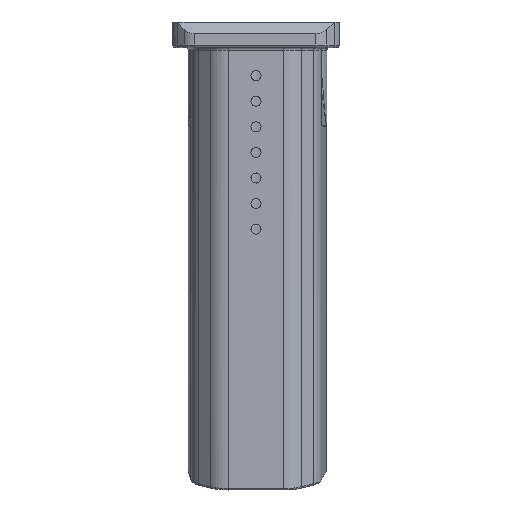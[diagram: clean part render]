
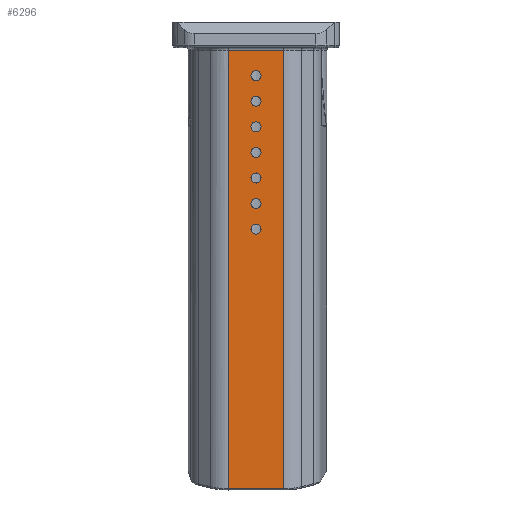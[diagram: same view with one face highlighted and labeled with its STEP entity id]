
A CAD part, front view. The second image highlights one B-rep face of the part: STEP entity #6296.
In plain terms, the highlighted planar face has unit normal (0, -1, 0).
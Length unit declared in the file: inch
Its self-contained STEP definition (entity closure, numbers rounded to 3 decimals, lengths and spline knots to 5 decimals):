
#50=FACE_BOUND('',#1745,.T.);
#51=FACE_BOUND('',#1746,.T.);
#52=FACE_BOUND('',#1747,.T.);
#53=FACE_BOUND('',#1748,.T.);
#54=FACE_BOUND('',#1749,.T.);
#55=FACE_BOUND('',#1750,.T.);
#56=FACE_BOUND('',#1751,.T.);
#136=PLANE('',#6984);
#452=LINE('',#13276,#797);
#485=LINE('',#13548,#830);
#486=LINE('',#13552,#831);
#515=LINE('',#14260,#860);
#797=VECTOR('',#8182,39.37008);
#830=VECTOR('',#8371,39.37008);
#831=VECTOR('',#8376,39.37008);
#860=VECTOR('',#8463,39.37008);
#1344=FACE_OUTER_BOUND('',#1744,.T.);
#1744=EDGE_LOOP('',(#5318,#5319,#5320,#5321));
#1745=EDGE_LOOP('',(#5322,#5323));
#1746=EDGE_LOOP('',(#5324,#5325));
#1747=EDGE_LOOP('',(#5326,#5327));
#1748=EDGE_LOOP('',(#5328,#5329));
#1749=EDGE_LOOP('',(#5330,#5331));
#1750=EDGE_LOOP('',(#5332,#5333));
#1751=EDGE_LOOP('',(#5334,#5335));
#2099=CIRCLE('',#6792,0.09843);
#2100=CIRCLE('',#6793,0.09843);
#2102=CIRCLE('',#6796,0.09843);
#2103=CIRCLE('',#6797,0.09843);
#2105=CIRCLE('',#6800,0.09843);
#2106=CIRCLE('',#6801,0.09843);
#2108=CIRCLE('',#6804,0.09843);
#2109=CIRCLE('',#6805,0.09843);
#2112=CIRCLE('',#6810,0.09843);
#2113=CIRCLE('',#6811,0.09843);
#2115=CIRCLE('',#6814,0.09843);
#2116=CIRCLE('',#6815,0.09843);
#2118=CIRCLE('',#6818,0.09843);
#2119=CIRCLE('',#6819,0.09843);
#2880=VERTEX_POINT('',#12572);
#2881=VERTEX_POINT('',#12573);
#2883=VERTEX_POINT('',#12580);
#2884=VERTEX_POINT('',#12581);
#2886=VERTEX_POINT('',#12588);
#2887=VERTEX_POINT('',#12589);
#2889=VERTEX_POINT('',#12596);
#2890=VERTEX_POINT('',#12597);
#2894=VERTEX_POINT('',#12608);
#2895=VERTEX_POINT('',#12609);
#2897=VERTEX_POINT('',#12616);
#2898=VERTEX_POINT('',#12617);
#2900=VERTEX_POINT('',#12624);
#2901=VERTEX_POINT('',#12625);
#2956=VERTEX_POINT('',#13272);
#2957=VERTEX_POINT('',#13274);
#3006=VERTEX_POINT('',#13546);
#3007=VERTEX_POINT('',#13551);
#3631=EDGE_CURVE('',#2880,#2881,#2099,.T.);
#3632=EDGE_CURVE('',#2881,#2880,#2100,.T.);
#3635=EDGE_CURVE('',#2883,#2884,#2102,.T.);
#3636=EDGE_CURVE('',#2884,#2883,#2103,.T.);
#3639=EDGE_CURVE('',#2886,#2887,#2105,.T.);
#3640=EDGE_CURVE('',#2887,#2886,#2106,.T.);
#3643=EDGE_CURVE('',#2889,#2890,#2108,.T.);
#3644=EDGE_CURVE('',#2890,#2889,#2109,.T.);
#3649=EDGE_CURVE('',#2894,#2895,#2112,.T.);
#3650=EDGE_CURVE('',#2895,#2894,#2113,.T.);
#3653=EDGE_CURVE('',#2897,#2898,#2115,.T.);
#3654=EDGE_CURVE('',#2898,#2897,#2116,.T.);
#3657=EDGE_CURVE('',#2900,#2901,#2118,.T.);
#3658=EDGE_CURVE('',#2901,#2900,#2119,.T.);
#3748=EDGE_CURVE('',#2957,#2956,#452,.T.);
#3836=EDGE_CURVE('',#2957,#3006,#485,.T.);
#3838=EDGE_CURVE('',#2956,#3007,#486,.T.);
#3894=EDGE_CURVE('',#3006,#3007,#515,.T.);
#5318=ORIENTED_EDGE('',*,*,#3836,.T.);
#5319=ORIENTED_EDGE('',*,*,#3894,.T.);
#5320=ORIENTED_EDGE('',*,*,#3838,.F.);
#5321=ORIENTED_EDGE('',*,*,#3748,.F.);
#5322=ORIENTED_EDGE('',*,*,#3631,.T.);
#5323=ORIENTED_EDGE('',*,*,#3632,.T.);
#5324=ORIENTED_EDGE('',*,*,#3635,.T.);
#5325=ORIENTED_EDGE('',*,*,#3636,.T.);
#5326=ORIENTED_EDGE('',*,*,#3639,.T.);
#5327=ORIENTED_EDGE('',*,*,#3640,.T.);
#5328=ORIENTED_EDGE('',*,*,#3643,.T.);
#5329=ORIENTED_EDGE('',*,*,#3644,.T.);
#5330=ORIENTED_EDGE('',*,*,#3649,.T.);
#5331=ORIENTED_EDGE('',*,*,#3650,.T.);
#5332=ORIENTED_EDGE('',*,*,#3653,.T.);
#5333=ORIENTED_EDGE('',*,*,#3654,.T.);
#5334=ORIENTED_EDGE('',*,*,#3657,.T.);
#5335=ORIENTED_EDGE('',*,*,#3658,.T.);
#6296=ADVANCED_FACE('',(#1344,#50,#51,#52,#53,#54,#55,#56),#136,.T.);
#6792=AXIS2_PLACEMENT_3D('',#12574,#7985,#7986);
#6793=AXIS2_PLACEMENT_3D('',#12575,#7987,#7988);
#6796=AXIS2_PLACEMENT_3D('',#12582,#7994,#7995);
#6797=AXIS2_PLACEMENT_3D('',#12583,#7996,#7997);
#6800=AXIS2_PLACEMENT_3D('',#12590,#8003,#8004);
#6801=AXIS2_PLACEMENT_3D('',#12591,#8005,#8006);
#6804=AXIS2_PLACEMENT_3D('',#12598,#8012,#8013);
#6805=AXIS2_PLACEMENT_3D('',#12599,#8014,#8015);
#6810=AXIS2_PLACEMENT_3D('',#12610,#8025,#8026);
#6811=AXIS2_PLACEMENT_3D('',#12611,#8027,#8028);
#6814=AXIS2_PLACEMENT_3D('',#12618,#8034,#8035);
#6815=AXIS2_PLACEMENT_3D('',#12619,#8036,#8037);
#6818=AXIS2_PLACEMENT_3D('',#12626,#8043,#8044);
#6819=AXIS2_PLACEMENT_3D('',#12627,#8045,#8046);
#6984=AXIS2_PLACEMENT_3D('',#14259,#8461,#8462);
#7985=DIRECTION('center_axis',(0.,1.,0.));
#7986=DIRECTION('ref_axis',(1.,0.,0.));
#7987=DIRECTION('center_axis',(0.,1.,0.));
#7988=DIRECTION('ref_axis',(1.,0.,0.));
#7994=DIRECTION('center_axis',(0.,1.,0.));
#7995=DIRECTION('ref_axis',(1.,0.,0.));
#7996=DIRECTION('center_axis',(0.,1.,0.));
#7997=DIRECTION('ref_axis',(1.,0.,0.));
#8003=DIRECTION('center_axis',(0.,1.,0.));
#8004=DIRECTION('ref_axis',(1.,0.,0.));
#8005=DIRECTION('center_axis',(0.,1.,0.));
#8006=DIRECTION('ref_axis',(1.,0.,0.));
#8012=DIRECTION('center_axis',(0.,1.,0.));
#8013=DIRECTION('ref_axis',(1.,0.,0.));
#8014=DIRECTION('center_axis',(0.,1.,0.));
#8015=DIRECTION('ref_axis',(1.,0.,0.));
#8025=DIRECTION('center_axis',(0.,1.,0.));
#8026=DIRECTION('ref_axis',(1.,0.,0.));
#8027=DIRECTION('center_axis',(0.,1.,0.));
#8028=DIRECTION('ref_axis',(1.,0.,0.));
#8034=DIRECTION('center_axis',(0.,1.,0.));
#8035=DIRECTION('ref_axis',(1.,0.,0.));
#8036=DIRECTION('center_axis',(0.,1.,0.));
#8037=DIRECTION('ref_axis',(1.,0.,0.));
#8043=DIRECTION('center_axis',(0.,1.,0.));
#8044=DIRECTION('ref_axis',(1.,0.,0.));
#8045=DIRECTION('center_axis',(0.,1.,0.));
#8046=DIRECTION('ref_axis',(1.,0.,0.));
#8182=DIRECTION('',(1.,0.,0.));
#8371=DIRECTION('',(0.,0.,-1.));
#8376=DIRECTION('',(0.,0.,-1.));
#8461=DIRECTION('center_axis',(0.,-1.,0.));
#8462=DIRECTION('ref_axis',(0.,0.,-1.));
#8463=DIRECTION('',(1.,0.,0.));
#12572=CARTESIAN_POINT('',(4.51516,-0.4932,-1.55));
#12573=CARTESIAN_POINT('',(4.31831,-0.4932,-1.55));
#12574=CARTESIAN_POINT('Origin',(4.41673,-0.4932,-1.55));
#12575=CARTESIAN_POINT('Origin',(4.41673,-0.4932,-1.55));
#12580=CARTESIAN_POINT('',(4.51516,-0.4932,-3.55));
#12581=CARTESIAN_POINT('',(4.31831,-0.4932,-3.55));
#12582=CARTESIAN_POINT('Origin',(4.41673,-0.4932,-3.55));
#12583=CARTESIAN_POINT('Origin',(4.41673,-0.4932,-3.55));
#12588=CARTESIAN_POINT('',(4.51516,-0.4932,-2.05));
#12589=CARTESIAN_POINT('',(4.31831,-0.4932,-2.05));
#12590=CARTESIAN_POINT('Origin',(4.41673,-0.4932,-2.05));
#12591=CARTESIAN_POINT('Origin',(4.41673,-0.4932,-2.05));
#12596=CARTESIAN_POINT('',(4.51516,-0.4932,-1.05));
#12597=CARTESIAN_POINT('',(4.31831,-0.4932,-1.05));
#12598=CARTESIAN_POINT('Origin',(4.41673,-0.4932,-1.05));
#12599=CARTESIAN_POINT('Origin',(4.41673,-0.4932,-1.05));
#12608=CARTESIAN_POINT('',(4.51516,-0.4932,-3.05));
#12609=CARTESIAN_POINT('',(4.31831,-0.4932,-3.05));
#12610=CARTESIAN_POINT('Origin',(4.41673,-0.4932,-3.05));
#12611=CARTESIAN_POINT('Origin',(4.41673,-0.4932,-3.05));
#12616=CARTESIAN_POINT('',(4.51516,-0.4932,-2.55));
#12617=CARTESIAN_POINT('',(4.31831,-0.4932,-2.55));
#12618=CARTESIAN_POINT('Origin',(4.41673,-0.4932,-2.55));
#12619=CARTESIAN_POINT('Origin',(4.41673,-0.4932,-2.55));
#12624=CARTESIAN_POINT('',(4.51516,-0.4932,-0.55));
#12625=CARTESIAN_POINT('',(4.31831,-0.4932,-0.55));
#12626=CARTESIAN_POINT('Origin',(4.41673,-0.4932,-0.55));
#12627=CARTESIAN_POINT('Origin',(4.41673,-0.4932,-0.55));
#13272=CARTESIAN_POINT('',(4.95505,-0.4932,-0.05));
#13274=CARTESIAN_POINT('',(3.87842,-0.4932,-0.05));
#13276=CARTESIAN_POINT('',(4.78942,-0.4932,-0.05));
#13546=CARTESIAN_POINT('',(3.87842,-0.4932,-8.62159));
#13548=CARTESIAN_POINT('',(3.87842,-0.4932,0.));
#13551=CARTESIAN_POINT('',(4.95505,-0.4932,-8.62159));
#13552=CARTESIAN_POINT('',(4.95505,-0.4932,0.));
#14259=CARTESIAN_POINT('Origin',(5.16216,-0.4932,0.));
#14260=CARTESIAN_POINT('',(5.16216,-0.4932,-8.62159));
